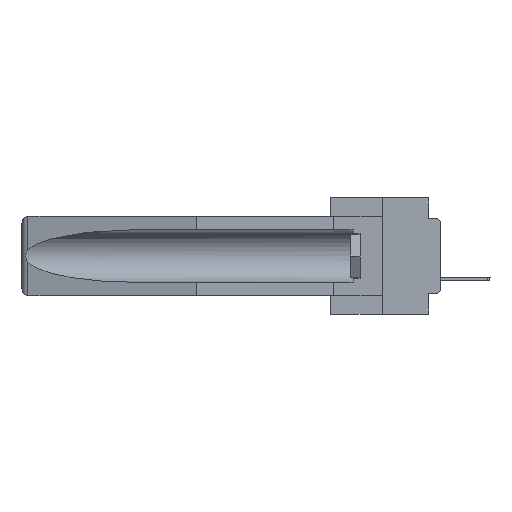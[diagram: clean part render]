
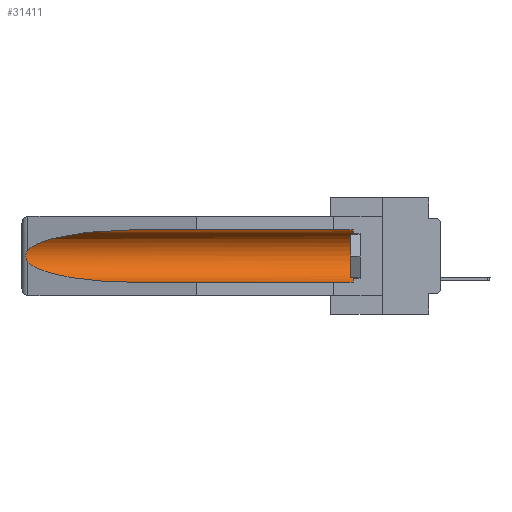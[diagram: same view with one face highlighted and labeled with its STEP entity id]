
A CAD part, left-side view. The second image highlights one B-rep face of the part: STEP entity #31411.
In plain terms, the highlighted cylindrical face has radius 2.857 mm (diameter 5.715 mm), a partial arc.
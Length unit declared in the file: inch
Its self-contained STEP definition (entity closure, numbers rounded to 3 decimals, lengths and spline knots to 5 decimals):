
#154 = ORIENTED_EDGE ( 'NONE', *, *, #7667, .T. ) ;
#572 = CARTESIAN_POINT ( 'NONE',  ( 0.21114, 1.30732, -0.059 ) ) ;
#2057 = CARTESIAN_POINT ( 'NONE',  ( 0.155, -0.30754, -0.1715 ) ) ;
#2245 = CARTESIAN_POINT ( 'NONE',  ( 0.155, 1.07973, -0.284 ) ) ;
#3673 = VERTEX_POINT ( 'NONE', #2245 ) ;
#3768 = EDGE_CURVE ( 'NONE', #13563, #3673, #33593, .T. ) ;
#4372 = EDGE_CURVE ( 'NONE', #5642, #3673, #10792, .T. ) ;
#5278 = CARTESIAN_POINT ( 'NONE',  ( 0.155, 0.126, -0.059 ) ) ;
#5364 = DIRECTION ( 'NONE',  ( 0., 1., 0. ) ) ;
#5642 = VERTEX_POINT ( 'NONE', #23739 ) ;
#7232 = CARTESIAN_POINT ( 'NONE',  ( 0.26597, 1.5296, -0.19026 ) ) ;
#7667 = EDGE_CURVE ( 'NONE', #26683, #30812, #11962, .T. ) ;
#8199 = ORIENTED_EDGE ( 'NONE', *, *, #35502, .T. ) ;
#8303 = DIRECTION ( 'NONE',  ( 0., 1., 0. ) ) ;
#8600 = VECTOR ( 'NONE', #5364, 39.37008 ) ;
#8840 = CARTESIAN_POINT ( 'NONE',  ( 0.25451, 1.48313, -0.09465 ) ) ;
#9004 = ORIENTED_EDGE ( 'NONE', *, *, #20013, .T. ) ;
#10166 = ORIENTED_EDGE ( 'NONE', *, *, #3768, .F. ) ;
#10792 =( BOUNDED_CURVE ( )  B_SPLINE_CURVE ( 3, ( #35294, #28867, #29414, #17686 ),
 .UNSPECIFIED., .F., .T. ) 
 B_SPLINE_CURVE_WITH_KNOTS ( ( 4, 4 ),
 ( 0.1948, 1.5708 ),
 .UNSPECIFIED. ) 
 CURVE ( )  GEOMETRIC_REPRESENTATION_ITEM ( )  RATIONAL_B_SPLINE_CURVE ( ( 1., 0.848, 0.848, 1. ) ) 
 REPRESENTATION_ITEM ( '' )  );
#10890 = EDGE_CURVE ( 'NONE', #17949, #26683, #28670, .T. ) ;
#11340 = B_SPLINE_CURVE_WITH_KNOTS ( 'NONE', 3,
 ( #26455, #12539, #12371, #17835, #34350, #23710, #15634, #34538, #7232, #20745 ),
 .UNSPECIFIED., .F., .F.,
 ( 4, 2, 2, 2, 4 ),
 ( 0., 0.00029, 0.00058, 0.00087, 0.00117 ),
 .UNSPECIFIED. ) ;
#11599 = CARTESIAN_POINT ( 'NONE',  ( 0.26537, 1.52718, -0.14972 ) ) ;
#11962 =( BOUNDED_CURVE ( )  B_SPLINE_CURVE ( 3, ( #30814, #572, #8840, #11599 ),
 .UNSPECIFIED., .F., .T. ) 
 B_SPLINE_CURVE_WITH_KNOTS ( ( 4, 4 ),
 ( 4.71239, 6.08839 ),
 .UNSPECIFIED. ) 
 CURVE ( )  GEOMETRIC_REPRESENTATION_ITEM ( )  RATIONAL_B_SPLINE_CURVE ( ( 1., 0.848, 0.848, 1. ) ) 
 REPRESENTATION_ITEM ( '' )  );
#12371 = CARTESIAN_POINT ( 'NONE',  ( 0.26654, 1.53092, -0.15636 ) ) ;
#12539 = CARTESIAN_POINT ( 'NONE',  ( 0.26597, 1.52961, -0.15275 ) ) ;
#13443 = DIRECTION ( 'NONE',  ( 0., 0., 1. ) ) ;
#13563 = VERTEX_POINT ( 'NONE', #14318 ) ;
#13964 = VECTOR ( 'NONE', #31796, 39.37008 ) ;
#14318 = CARTESIAN_POINT ( 'NONE',  ( 0.155, 0.126, -0.284 ) ) ;
#15588 = AXIS2_PLACEMENT_3D ( 'NONE', #18579, #15650, #18033 ) ;
#15634 = CARTESIAN_POINT ( 'NONE',  ( 0.2673, 1.53269, -0.17917 ) ) ;
#15650 = DIRECTION ( 'NONE',  ( 0., -1., 0. ) ) ;
#16761 = CIRCLE ( 'NONE', #15588, 0.1125 ) ;
#17686 = CARTESIAN_POINT ( 'NONE',  ( 0.155, 1.07973, -0.284 ) ) ;
#17835 = CARTESIAN_POINT ( 'NONE',  ( 0.2673, 1.5327, -0.16383 ) ) ;
#17949 = VERTEX_POINT ( 'NONE', #5278 ) ;
#18033 = DIRECTION ( 'NONE',  ( 0., 0., 1. ) ) ;
#18579 = CARTESIAN_POINT ( 'NONE',  ( 0.155, 0.126, -0.1715 ) ) ;
#20013 = EDGE_CURVE ( 'NONE', #30812, #5642, #11340, .T. ) ;
#20745 = CARTESIAN_POINT ( 'NONE',  ( 0.26537, 1.52718, -0.19328 ) ) ;
#23013 = CARTESIAN_POINT ( 'NONE',  ( 0.155, -0.30754, -0.059 ) ) ;
#23406 = ORIENTED_EDGE ( 'NONE', *, *, #4372, .T. ) ;
#23543 = ORIENTED_EDGE ( 'NONE', *, *, #10890, .T. ) ;
#23710 = CARTESIAN_POINT ( 'NONE',  ( 0.2675, 1.53308, -0.17534 ) ) ;
#23739 = CARTESIAN_POINT ( 'NONE',  ( 0.26537, 1.52718, -0.19328 ) ) ;
#24961 = CYLINDRICAL_SURFACE ( 'NONE', #28812, 0.1125 ) ;
#25140 = CARTESIAN_POINT ( 'NONE',  ( 0.155, -0.30754, -0.284 ) ) ;
#26455 = CARTESIAN_POINT ( 'NONE',  ( 0.26537, 1.52718, -0.14972 ) ) ;
#26486 = CARTESIAN_POINT ( 'NONE',  ( 0.26537, 1.52718, -0.14972 ) ) ;
#26683 = VERTEX_POINT ( 'NONE', #27265 ) ;
#27265 = CARTESIAN_POINT ( 'NONE',  ( 0.155, 1.07973, -0.059 ) ) ;
#28349 = EDGE_LOOP ( 'NONE', ( #154, #9004, #23406, #10166, #8199, #23543 ) ) ;
#28670 = LINE ( 'NONE', #23013, #13964 ) ;
#28812 = AXIS2_PLACEMENT_3D ( 'NONE', #2057, #8303, #13443 ) ;
#28867 = CARTESIAN_POINT ( 'NONE',  ( 0.25451, 1.48313, -0.24835 ) ) ;
#29414 = CARTESIAN_POINT ( 'NONE',  ( 0.21114, 1.30732, -0.284 ) ) ;
#30812 = VERTEX_POINT ( 'NONE', #26486 ) ;
#30814 = CARTESIAN_POINT ( 'NONE',  ( 0.155, 1.07973, -0.059 ) ) ;
#31411 = ADVANCED_FACE ( 'NONE', ( #32681 ), #24961, .F. ) ;
#31796 = DIRECTION ( 'NONE',  ( 0., 1., 0. ) ) ;
#32681 = FACE_OUTER_BOUND ( 'NONE', #28349, .T. ) ;
#33593 = LINE ( 'NONE', #25140, #8600 ) ;
#34350 = CARTESIAN_POINT ( 'NONE',  ( 0.2675, 1.53308, -0.16763 ) ) ;
#34538 = CARTESIAN_POINT ( 'NONE',  ( 0.26655, 1.53094, -0.18657 ) ) ;
#35294 = CARTESIAN_POINT ( 'NONE',  ( 0.26537, 1.52718, -0.19328 ) ) ;
#35502 = EDGE_CURVE ( 'NONE', #13563, #17949, #16761, .T. ) ;
